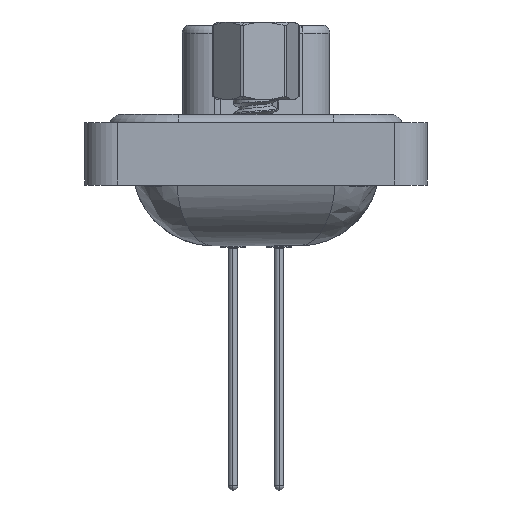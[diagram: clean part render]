
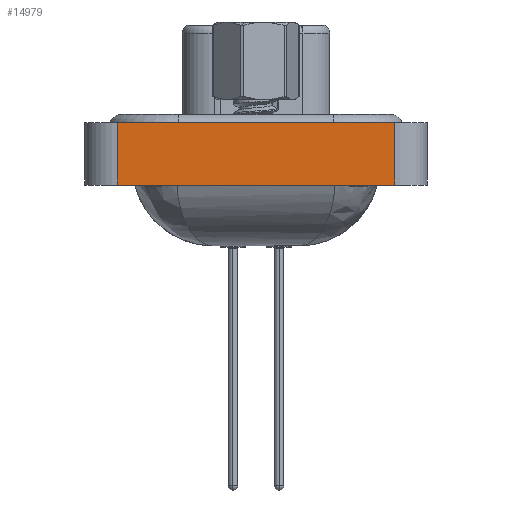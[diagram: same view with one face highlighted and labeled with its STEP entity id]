
A CAD part, left-side view. The second image highlights one B-rep face of the part: STEP entity #14979.
In plain terms, the highlighted planar face has unit normal (-1, 0, 0).
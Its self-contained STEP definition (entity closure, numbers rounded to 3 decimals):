
#111 = ORIENTED_EDGE ( 'NONE', *, *, #4300, .T. ) ;
#884 = LINE ( 'NONE', #3225, #7466 ) ;
#1192 = VECTOR ( 'NONE', #5455, 1000. ) ;
#3068 = ORIENTED_EDGE ( 'NONE', *, *, #14817, .F. ) ;
#3225 = CARTESIAN_POINT ( 'NONE',  ( -7.15, 8.55, -3.35 ) ) ;
#3306 = LINE ( 'NONE', #7796, #1192 ) ;
#4022 = CARTESIAN_POINT ( 'NONE',  ( -7.15, 8.55, -3.35 ) ) ;
#4040 = DIRECTION ( 'NONE',  ( 0., 0., 1. ) ) ;
#4300 = EDGE_CURVE ( 'NONE', #28575, #14113, #6287, .T. ) ;
#5455 = DIRECTION ( 'NONE',  ( 0., -1., 0. ) ) ;
#6287 = LINE ( 'NONE', #31883, #19250 ) ;
#7466 = VECTOR ( 'NONE', #18065, 1000. ) ;
#7490 = DIRECTION ( 'NONE',  ( 0., -1., 0. ) ) ;
#7796 = CARTESIAN_POINT ( 'NONE',  ( -7.15, -8.55, 0.5 ) ) ;
#9061 = AXIS2_PLACEMENT_3D ( 'NONE', #11566, #18901, #4040 ) ;
#9858 = VERTEX_POINT ( 'NONE', #4022 ) ;
#11566 = CARTESIAN_POINT ( 'NONE',  ( -7.15, -8.55, -3.35 ) ) ;
#12444 = CARTESIAN_POINT ( 'NONE',  ( -7.15, -8.55, -3.35 ) ) ;
#14113 = VERTEX_POINT ( 'NONE', #16352 ) ;
#14817 = EDGE_CURVE ( 'NONE', #9858, #19836, #884, .T. ) ;
#14850 = CARTESIAN_POINT ( 'NONE',  ( -7.15, -8.55, -3.35 ) ) ;
#14979 = ADVANCED_FACE ( 'NONE', ( #24261 ), #29781, .T. ) ;
#16352 = CARTESIAN_POINT ( 'NONE',  ( -7.15, -8.55, 0.5 ) ) ;
#17050 = EDGE_CURVE ( 'NONE', #19836, #14113, #3306, .T. ) ;
#18065 = DIRECTION ( 'NONE',  ( 0., 0., 1. ) ) ;
#18901 = DIRECTION ( 'NONE',  ( -1., 0., 0. ) ) ;
#19250 = VECTOR ( 'NONE', #19795, 1000. ) ;
#19795 = DIRECTION ( 'NONE',  ( 0., 0., 1. ) ) ;
#19836 = VERTEX_POINT ( 'NONE', #20917 ) ;
#20917 = CARTESIAN_POINT ( 'NONE',  ( -7.15, 8.55, 0.5 ) ) ;
#20949 = VECTOR ( 'NONE', #7490, 1000. ) ;
#22253 = ORIENTED_EDGE ( 'NONE', *, *, #17050, .F. ) ;
#24261 = FACE_OUTER_BOUND ( 'NONE', #30441, .T. ) ;
#25528 = LINE ( 'NONE', #14850, #20949 ) ;
#28575 = VERTEX_POINT ( 'NONE', #12444 ) ;
#29201 = EDGE_CURVE ( 'NONE', #9858, #28575, #25528, .T. ) ;
#29781 = PLANE ( 'NONE',  #9061 ) ;
#30362 = ORIENTED_EDGE ( 'NONE', *, *, #29201, .T. ) ;
#30441 = EDGE_LOOP ( 'NONE', ( #111, #22253, #3068, #30362 ) ) ;
#31883 = CARTESIAN_POINT ( 'NONE',  ( -7.15, -8.55, -3.35 ) ) ;
